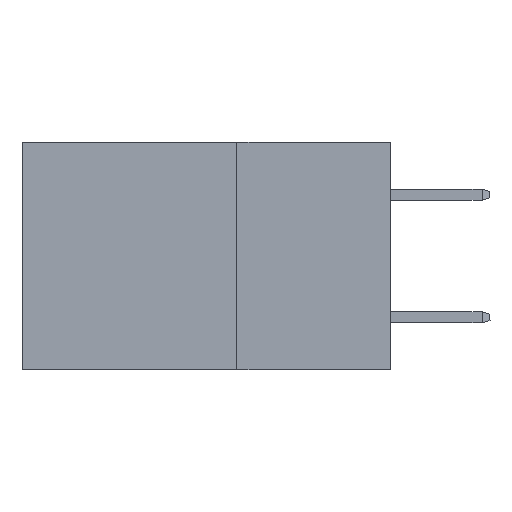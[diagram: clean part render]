
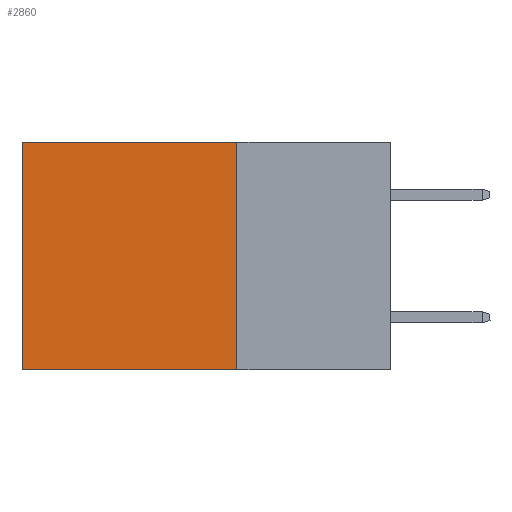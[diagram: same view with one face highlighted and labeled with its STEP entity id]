
A CAD part, left-side view. The second image highlights one B-rep face of the part: STEP entity #2860.
In plain terms, the highlighted planar face has unit normal (-1, 0, 0).
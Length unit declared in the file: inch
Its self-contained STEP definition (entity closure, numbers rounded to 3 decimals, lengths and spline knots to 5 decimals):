
#664 = CARTESIAN_POINT ( 'NONE',  ( 0.2875, 0.25, -0.37 ) ) ;
#1371 = LINE ( 'NONE', #4936, #4932 ) ;
#2102 = DIRECTION ( 'NONE',  ( 0., 0., -1. ) ) ;
#2368 = CARTESIAN_POINT ( 'NONE',  ( 0.2875, 0.6, -0.37 ) ) ;
#2860 = ADVANCED_FACE ( 'NONE', ( #13337 ), #11464, .F. ) ;
#2942 = VERTEX_POINT ( 'NONE', #18925 ) ;
#3971 = CARTESIAN_POINT ( 'NONE',  ( 0.2875, 0.25, 0. ) ) ;
#4013 = VERTEX_POINT ( 'NONE', #6517 ) ;
#4932 = VECTOR ( 'NONE', #12399, 39.37008 ) ;
#4936 = CARTESIAN_POINT ( 'NONE',  ( 0.2875, 0.25, 0. ) ) ;
#5498 = DIRECTION ( 'NONE',  ( 0., 0., -1. ) ) ;
#5916 = ORIENTED_EDGE ( 'NONE', *, *, #13213, .F. ) ;
#6135 = ORIENTED_EDGE ( 'NONE', *, *, #12885, .T. ) ;
#6517 = CARTESIAN_POINT ( 'NONE',  ( 0.2875, 0.6, 0. ) ) ;
#6997 = DIRECTION ( 'NONE',  ( 0., 1., 0. ) ) ;
#7707 = DIRECTION ( 'NONE',  ( 0., 1., 0. ) ) ;
#8932 = VECTOR ( 'NONE', #2102, 39.37008 ) ;
#9409 = LINE ( 'NONE', #9627, #8932 ) ;
#9627 = CARTESIAN_POINT ( 'NONE',  ( 0.2875, 0.6, 0. ) ) ;
#10397 = LINE ( 'NONE', #12924, #17671 ) ;
#10826 = VERTEX_POINT ( 'NONE', #2368 ) ;
#11464 = PLANE ( 'NONE',  #17331 ) ;
#12399 = DIRECTION ( 'NONE',  ( 0., 0., -1. ) ) ;
#12611 = ORIENTED_EDGE ( 'NONE', *, *, #14179, .T. ) ;
#12885 = EDGE_CURVE ( 'NONE', #2942, #4013, #18608, .T. ) ;
#12924 = CARTESIAN_POINT ( 'NONE',  ( 0.2875, 0.25, -0.37 ) ) ;
#13213 = EDGE_CURVE ( 'NONE', #18932, #10826, #10397, .T. ) ;
#13337 = FACE_OUTER_BOUND ( 'NONE', #15110, .T. ) ;
#13504 = ORIENTED_EDGE ( 'NONE', *, *, #16596, .F. ) ;
#14179 = EDGE_CURVE ( 'NONE', #4013, #10826, #9409, .T. ) ;
#14418 = DIRECTION ( 'NONE',  ( 1., 0., 0. ) ) ;
#15110 = EDGE_LOOP ( 'NONE', ( #12611, #5916, #13504, #6135 ) ) ;
#16506 = CARTESIAN_POINT ( 'NONE',  ( 0.2875, 0.25, 0. ) ) ;
#16596 = EDGE_CURVE ( 'NONE', #2942, #18932, #1371, .T. ) ;
#17331 = AXIS2_PLACEMENT_3D ( 'NONE', #3971, #14418, #5498 ) ;
#17671 = VECTOR ( 'NONE', #6997, 39.37008 ) ;
#18140 = VECTOR ( 'NONE', #7707, 39.37008 ) ;
#18608 = LINE ( 'NONE', #16506, #18140 ) ;
#18925 = CARTESIAN_POINT ( 'NONE',  ( 0.2875, 0.25, 0. ) ) ;
#18932 = VERTEX_POINT ( 'NONE', #664 ) ;
